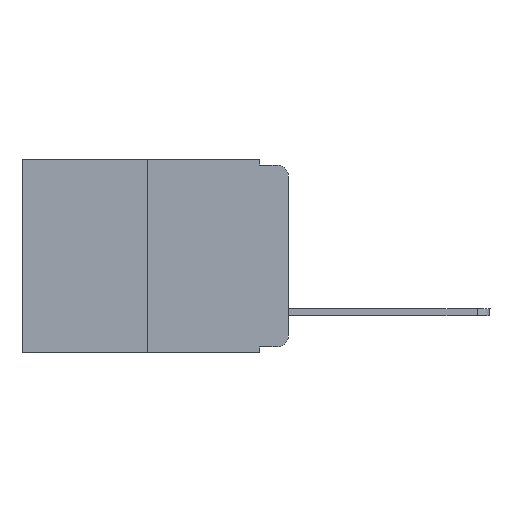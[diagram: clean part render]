
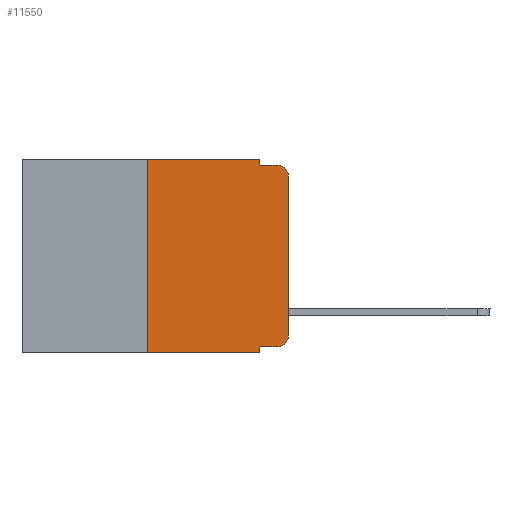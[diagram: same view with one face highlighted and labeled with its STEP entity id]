
A CAD part, left-side view. The second image highlights one B-rep face of the part: STEP entity #11550.
In plain terms, the highlighted planar face has unit normal (-1, 0, 0).
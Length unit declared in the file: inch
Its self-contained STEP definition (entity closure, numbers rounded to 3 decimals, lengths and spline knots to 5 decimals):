
#247 = DIRECTION ( 'NONE',  ( -1., 0., 0. ) ) ;
#367 = EDGE_CURVE ( 'NONE', #4941, #4882, #1826, .T. ) ;
#716 = LINE ( 'NONE', #4379, #1869 ) ;
#977 = VECTOR ( 'NONE', #2033, 39.37008 ) ;
#1062 = CARTESIAN_POINT ( 'NONE',  ( 0., 0., -0.03 ) ) ;
#1066 = VERTEX_POINT ( 'NONE', #9961 ) ;
#1103 = CIRCLE ( 'NONE', #7186, 0.02 ) ;
#1187 = LINE ( 'NONE', #1235, #977 ) ;
#1235 = CARTESIAN_POINT ( 'NONE',  ( 0., 0.473, -0.343 ) ) ;
#1458 = ORIENTED_EDGE ( 'NONE', *, *, #3370, .T. ) ;
#1636 = EDGE_CURVE ( 'NONE', #8451, #7225, #11023, .T. ) ;
#1826 = CIRCLE ( 'NONE', #4869, 0.02 ) ;
#1869 = VECTOR ( 'NONE', #3033, 39.37008 ) ;
#2033 = DIRECTION ( 'NONE',  ( 0., -1., 0. ) ) ;
#2104 = CARTESIAN_POINT ( 'NONE',  ( 0., 0., -0.313 ) ) ;
#2343 = VECTOR ( 'NONE', #10505, 39.37008 ) ;
#2642 = LINE ( 'NONE', #9717, #3864 ) ;
#2655 = ORIENTED_EDGE ( 'NONE', *, *, #10107, .F. ) ;
#2682 = CARTESIAN_POINT ( 'NONE',  ( 0., 0.051, -0.01 ) ) ;
#2867 = CARTESIAN_POINT ( 'NONE',  ( 0., 0.473, 0. ) ) ;
#2992 = DIRECTION ( 'NONE',  ( 0., -1., 0. ) ) ;
#3002 = DIRECTION ( 'NONE',  ( 1., 0., 0. ) ) ;
#3033 = DIRECTION ( 'NONE',  ( 0., -1., 0. ) ) ;
#3370 = EDGE_CURVE ( 'NONE', #1066, #7819, #1187, .T. ) ;
#3391 = VECTOR ( 'NONE', #2992, 39.37008 ) ;
#3463 = EDGE_CURVE ( 'NONE', #1066, #8451, #6610, .T. ) ;
#3652 = VECTOR ( 'NONE', #8716, 39.37008 ) ;
#3708 = EDGE_CURVE ( 'NONE', #10304, #5928, #1103, .T. ) ;
#3864 = VECTOR ( 'NONE', #8772, 39.37008 ) ;
#3912 = PLANE ( 'NONE',  #10089 ) ;
#4124 = DIRECTION ( 'NONE',  ( 0., 0., -1. ) ) ;
#4198 = CARTESIAN_POINT ( 'NONE',  ( 0., 0.02, -0.01 ) ) ;
#4379 = CARTESIAN_POINT ( 'NONE',  ( 0., 0.051, -0.01 ) ) ;
#4424 = CARTESIAN_POINT ( 'NONE',  ( 0., 0.051, 0. ) ) ;
#4869 = AXIS2_PLACEMENT_3D ( 'NONE', #11199, #247, #5691 ) ;
#4882 = VERTEX_POINT ( 'NONE', #4198 ) ;
#4941 = VERTEX_POINT ( 'NONE', #1062 ) ;
#5045 = CARTESIAN_POINT ( 'NONE',  ( 0., 0.051, 0. ) ) ;
#5263 = ORIENTED_EDGE ( 'NONE', *, *, #367, .T. ) ;
#5315 = EDGE_CURVE ( 'NONE', #5928, #4941, #11403, .T. ) ;
#5691 = DIRECTION ( 'NONE',  ( 0., 0., -1. ) ) ;
#5740 = CARTESIAN_POINT ( 'NONE',  ( 0., 0.25, 0. ) ) ;
#5835 = CARTESIAN_POINT ( 'NONE',  ( 0., 0.25, 0. ) ) ;
#5928 = VERTEX_POINT ( 'NONE', #2104 ) ;
#6080 = CARTESIAN_POINT ( 'NONE',  ( 0., 0.051, -0.343 ) ) ;
#6304 = VERTEX_POINT ( 'NONE', #6374 ) ;
#6374 = CARTESIAN_POINT ( 'NONE',  ( 0., 0.051, -0.333 ) ) ;
#6423 = DIRECTION ( 'NONE',  ( 0., 0., -1. ) ) ;
#6610 = LINE ( 'NONE', #5835, #7433 ) ;
#6859 = ORIENTED_EDGE ( 'NONE', *, *, #3708, .T. ) ;
#6896 = CARTESIAN_POINT ( 'NONE',  ( 0., 0., 0. ) ) ;
#6932 = ORIENTED_EDGE ( 'NONE', *, *, #3463, .F. ) ;
#7186 = AXIS2_PLACEMENT_3D ( 'NONE', #8961, #7314, #10753 ) ;
#7225 = VERTEX_POINT ( 'NONE', #7472 ) ;
#7268 = ORIENTED_EDGE ( 'NONE', *, *, #11625, .F. ) ;
#7314 = DIRECTION ( 'NONE',  ( -1., 0., 0. ) ) ;
#7433 = VECTOR ( 'NONE', #11190, 39.37008 ) ;
#7472 = CARTESIAN_POINT ( 'NONE',  ( 0., 0.051, 0. ) ) ;
#7819 = VERTEX_POINT ( 'NONE', #6080 ) ;
#8252 = EDGE_LOOP ( 'NONE', ( #10067, #5263, #2655, #7268, #8757, #6932, #1458, #10047, #8902, #6859 ) ) ;
#8451 = VERTEX_POINT ( 'NONE', #5740 ) ;
#8716 = DIRECTION ( 'NONE',  ( 0., 0., -1. ) ) ;
#8757 = ORIENTED_EDGE ( 'NONE', *, *, #1636, .F. ) ;
#8772 = DIRECTION ( 'NONE',  ( 0., -1., 0. ) ) ;
#8796 = CARTESIAN_POINT ( 'NONE',  ( 0., 0.02, -0.333 ) ) ;
#8902 = ORIENTED_EDGE ( 'NONE', *, *, #11307, .T. ) ;
#8916 = LINE ( 'NONE', #4424, #9346 ) ;
#8961 = CARTESIAN_POINT ( 'NONE',  ( 0., 0.02, -0.313 ) ) ;
#9346 = VECTOR ( 'NONE', #6423, 39.37008 ) ;
#9425 = LINE ( 'NONE', #5045, #3652 ) ;
#9717 = CARTESIAN_POINT ( 'NONE',  ( 0., 0.051, -0.333 ) ) ;
#9961 = CARTESIAN_POINT ( 'NONE',  ( 0., 0.25, -0.343 ) ) ;
#10002 = VERTEX_POINT ( 'NONE', #2682 ) ;
#10047 = ORIENTED_EDGE ( 'NONE', *, *, #11174, .F. ) ;
#10067 = ORIENTED_EDGE ( 'NONE', *, *, #5315, .T. ) ;
#10089 = AXIS2_PLACEMENT_3D ( 'NONE', #11418, #3002, #4124 ) ;
#10107 = EDGE_CURVE ( 'NONE', #10002, #4882, #716, .T. ) ;
#10304 = VERTEX_POINT ( 'NONE', #8796 ) ;
#10505 = DIRECTION ( 'NONE',  ( 0., 0., 1. ) ) ;
#10753 = DIRECTION ( 'NONE',  ( 0., 0., -1. ) ) ;
#11023 = LINE ( 'NONE', #2867, #3391 ) ;
#11174 = EDGE_CURVE ( 'NONE', #6304, #7819, #9425, .T. ) ;
#11190 = DIRECTION ( 'NONE',  ( 0., 0., 1. ) ) ;
#11199 = CARTESIAN_POINT ( 'NONE',  ( 0., 0.02, -0.03 ) ) ;
#11307 = EDGE_CURVE ( 'NONE', #6304, #10304, #2642, .T. ) ;
#11403 = LINE ( 'NONE', #6896, #2343 ) ;
#11418 = CARTESIAN_POINT ( 'NONE',  ( 0., 0.473, 0. ) ) ;
#11539 = FACE_OUTER_BOUND ( 'NONE', #8252, .T. ) ;
#11550 = ADVANCED_FACE ( 'NONE', ( #11539 ), #3912, .F. ) ;
#11625 = EDGE_CURVE ( 'NONE', #7225, #10002, #8916, .T. ) ;
